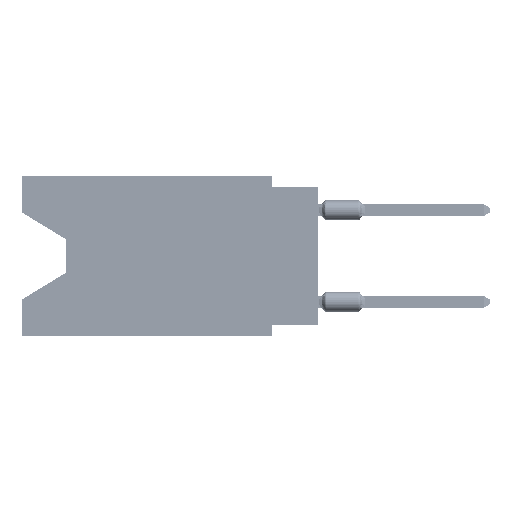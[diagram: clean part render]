
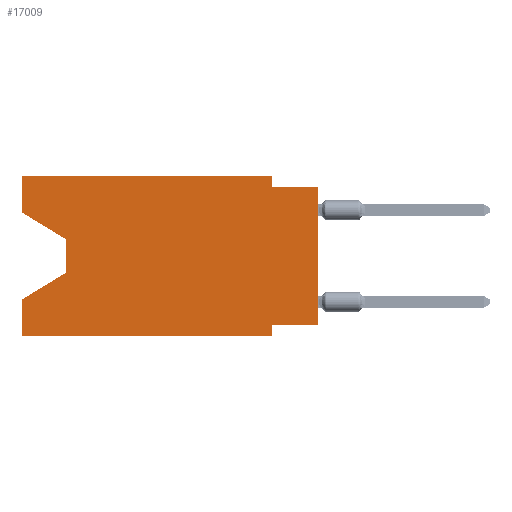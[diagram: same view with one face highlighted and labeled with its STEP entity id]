
A CAD part, left-side view. The second image highlights one B-rep face of the part: STEP entity #17009.
In plain terms, the highlighted planar face has unit normal (-1, 0, 0).
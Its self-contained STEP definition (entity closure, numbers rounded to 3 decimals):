
#412 = VECTOR ( 'NONE', #2762, 1000. ) ;
#1037 = CARTESIAN_POINT ( 'NONE',  ( 0., 0., -8.255 ) ) ;
#1767 = DIRECTION ( 'NONE',  ( 0., 0., -1. ) ) ;
#2762 = DIRECTION ( 'NONE',  ( 0., 0., 1. ) ) ;
#3240 = VECTOR ( 'NONE', #10021, 1000. ) ;
#5331 = LINE ( 'NONE', #6652, #42613 ) ;
#5857 = CARTESIAN_POINT ( 'NONE',  ( 0., 16.383, -2.038 ) ) ;
#6649 = VECTOR ( 'NONE', #13527, 1000. ) ;
#6652 = CARTESIAN_POINT ( 'NONE',  ( 0., 13.97, -5.385 ) ) ;
#6814 = VERTEX_POINT ( 'NONE', #33792 ) ;
#6912 = CARTESIAN_POINT ( 'NONE',  ( 0., 2.54, -0.635 ) ) ;
#6921 = ORIENTED_EDGE ( 'NONE', *, *, #54747, .F. ) ;
#6926 = CARTESIAN_POINT ( 'NONE',  ( 0., 13.97, -3.505 ) ) ;
#7536 = CARTESIAN_POINT ( 'NONE',  ( 0., 0., -8.255 ) ) ;
#7628 = DIRECTION ( 'NONE',  ( 0., 0., -1. ) ) ;
#8189 = LINE ( 'NONE', #28586, #47198 ) ;
#8774 = DIRECTION ( 'NONE',  ( 0., 0., -1. ) ) ;
#8835 = EDGE_CURVE ( 'NONE', #6814, #12063, #17819, .T. ) ;
#9149 = VERTEX_POINT ( 'NONE', #1037 ) ;
#9405 = CARTESIAN_POINT ( 'NONE',  ( 0., 16.383, 0. ) ) ;
#9428 = VERTEX_POINT ( 'NONE', #24978 ) ;
#9486 = VECTOR ( 'NONE', #12035, 1000. ) ;
#10021 = DIRECTION ( 'NONE',  ( 0., -1., 0. ) ) ;
#10501 = ORIENTED_EDGE ( 'NONE', *, *, #49132, .T. ) ;
#10762 = ORIENTED_EDGE ( 'NONE', *, *, #12344, .T. ) ;
#10881 = LINE ( 'NONE', #5857, #30499 ) ;
#11456 = CARTESIAN_POINT ( 'NONE',  ( 0., 13.97, -5.385 ) ) ;
#12035 = DIRECTION ( 'NONE',  ( 0., -1., 0. ) ) ;
#12063 = VERTEX_POINT ( 'NONE', #13066 ) ;
#12344 = EDGE_CURVE ( 'NONE', #28942, #12063, #5331, .T. ) ;
#13066 = CARTESIAN_POINT ( 'NONE',  ( 0., 16.383, -6.852 ) ) ;
#13261 = CARTESIAN_POINT ( 'NONE',  ( 0., 0., -0.635 ) ) ;
#13527 = DIRECTION ( 'NONE',  ( 0., 1., 0. ) ) ;
#13818 = DIRECTION ( 'NONE',  ( 0., -1., 0. ) ) ;
#14202 = VERTEX_POINT ( 'NONE', #6912 ) ;
#14903 = CARTESIAN_POINT ( 'NONE',  ( 0., 2.54, -8.89 ) ) ;
#15044 = LINE ( 'NONE', #61191, #3240 ) ;
#15996 = VECTOR ( 'NONE', #7628, 1000. ) ;
#16414 = EDGE_CURVE ( 'NONE', #9149, #9428, #23225, .T. ) ;
#16572 = VECTOR ( 'NONE', #1767, 1000. ) ;
#17007 = VERTEX_POINT ( 'NONE', #39185 ) ;
#17009 = ADVANCED_FACE ( 'NONE', ( #49237 ), #20102, .F. ) ;
#17052 = LINE ( 'NONE', #58185, #9486 ) ;
#17819 = LINE ( 'NONE', #52934, #412 ) ;
#17979 = LINE ( 'NONE', #22672, #15996 ) ;
#18434 = AXIS2_PLACEMENT_3D ( 'NONE', #9405, #30138, #8774 ) ;
#19864 = EDGE_CURVE ( 'NONE', #9428, #45549, #38205, .T. ) ;
#20102 = PLANE ( 'NONE',  #18434 ) ;
#20983 = DIRECTION ( 'NONE',  ( 0., 0., -1. ) ) ;
#22193 = EDGE_LOOP ( 'NONE', ( #50807, #10501, #10762, #31447, #47659, #23842, #50484, #44207, #6921, #64291, #59620, #50478 ) ) ;
#22672 = CARTESIAN_POINT ( 'NONE',  ( 0., 2.54, 0. ) ) ;
#23225 = LINE ( 'NONE', #7536, #6649 ) ;
#23842 = ORIENTED_EDGE ( 'NONE', *, *, #19864, .F. ) ;
#24978 = CARTESIAN_POINT ( 'NONE',  ( 0., 2.54, -8.255 ) ) ;
#25068 = VECTOR ( 'NONE', #13818, 1000. ) ;
#26372 = CARTESIAN_POINT ( 'NONE',  ( 0., 16.383, -2.038 ) ) ;
#26402 = LINE ( 'NONE', #30750, #65684 ) ;
#28586 = CARTESIAN_POINT ( 'NONE',  ( 0., 0., 0. ) ) ;
#28942 = VERTEX_POINT ( 'NONE', #11456 ) ;
#29332 = VERTEX_POINT ( 'NONE', #46816 ) ;
#30138 = DIRECTION ( 'NONE',  ( 1., 0., 0. ) ) ;
#30499 = VECTOR ( 'NONE', #62027, 1000. ) ;
#30750 = CARTESIAN_POINT ( 'NONE',  ( 0., 16.383, 0. ) ) ;
#31060 = VERTEX_POINT ( 'NONE', #13261 ) ;
#31447 = ORIENTED_EDGE ( 'NONE', *, *, #8835, .F. ) ;
#32873 = EDGE_CURVE ( 'NONE', #9149, #31060, #8189, .T. ) ;
#33693 = VECTOR ( 'NONE', #20983, 1000. ) ;
#33792 = CARTESIAN_POINT ( 'NONE',  ( 0., 16.383, -8.89 ) ) ;
#38205 = LINE ( 'NONE', #52264, #16572 ) ;
#39185 = CARTESIAN_POINT ( 'NONE',  ( 0., 13.97, -3.505 ) ) ;
#41120 = LINE ( 'NONE', #59974, #25068 ) ;
#42613 = VECTOR ( 'NONE', #47428, 1000. ) ;
#44207 = ORIENTED_EDGE ( 'NONE', *, *, #32873, .T. ) ;
#45549 = VERTEX_POINT ( 'NONE', #14903 ) ;
#46816 = CARTESIAN_POINT ( 'NONE',  ( 0., 16.383, 0. ) ) ;
#47198 = VECTOR ( 'NONE', #59352, 1000. ) ;
#47428 = DIRECTION ( 'NONE',  ( 0., 0.855, -0.519 ) ) ;
#47659 = ORIENTED_EDGE ( 'NONE', *, *, #64120, .T. ) ;
#49132 = EDGE_CURVE ( 'NONE', #17007, #28942, #51436, .T. ) ;
#49237 = FACE_OUTER_BOUND ( 'NONE', #22193, .T. ) ;
#50478 = ORIENTED_EDGE ( 'NONE', *, *, #62441, .F. ) ;
#50484 = ORIENTED_EDGE ( 'NONE', *, *, #16414, .F. ) ;
#50807 = ORIENTED_EDGE ( 'NONE', *, *, #65142, .T. ) ;
#51163 = DIRECTION ( 'NONE',  ( 0., 0., 1. ) ) ;
#51436 = LINE ( 'NONE', #6926, #33693 ) ;
#52264 = CARTESIAN_POINT ( 'NONE',  ( 0., 2.54, -8.89 ) ) ;
#52934 = CARTESIAN_POINT ( 'NONE',  ( 0., 16.383, 0. ) ) ;
#54747 = EDGE_CURVE ( 'NONE', #14202, #31060, #17052, .T. ) ;
#55720 = EDGE_CURVE ( 'NONE', #56597, #14202, #17979, .T. ) ;
#56597 = VERTEX_POINT ( 'NONE', #62312 ) ;
#57334 = VERTEX_POINT ( 'NONE', #26372 ) ;
#58185 = CARTESIAN_POINT ( 'NONE',  ( 0., 0., -0.635 ) ) ;
#58483 = EDGE_CURVE ( 'NONE', #29332, #56597, #15044, .T. ) ;
#59352 = DIRECTION ( 'NONE',  ( 0., 0., 1. ) ) ;
#59620 = ORIENTED_EDGE ( 'NONE', *, *, #58483, .F. ) ;
#59974 = CARTESIAN_POINT ( 'NONE',  ( 0., 16.383, -8.89 ) ) ;
#61191 = CARTESIAN_POINT ( 'NONE',  ( 0., 16.383, 0. ) ) ;
#62027 = DIRECTION ( 'NONE',  ( 0., -0.855, -0.519 ) ) ;
#62312 = CARTESIAN_POINT ( 'NONE',  ( 0., 2.54, 0. ) ) ;
#62441 = EDGE_CURVE ( 'NONE', #57334, #29332, #26402, .T. ) ;
#64120 = EDGE_CURVE ( 'NONE', #6814, #45549, #41120, .T. ) ;
#64291 = ORIENTED_EDGE ( 'NONE', *, *, #55720, .F. ) ;
#65142 = EDGE_CURVE ( 'NONE', #57334, #17007, #10881, .T. ) ;
#65684 = VECTOR ( 'NONE', #51163, 1000. ) ;
